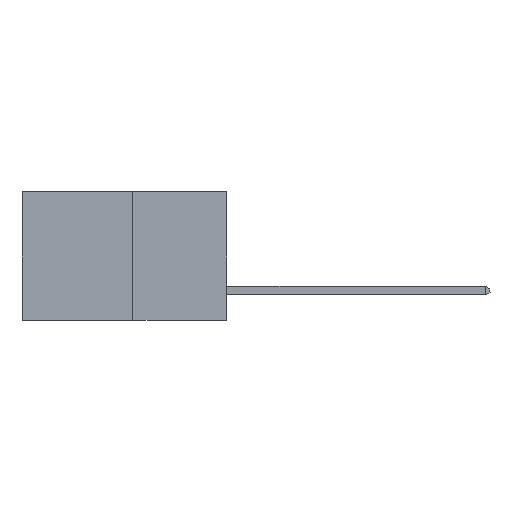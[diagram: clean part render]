
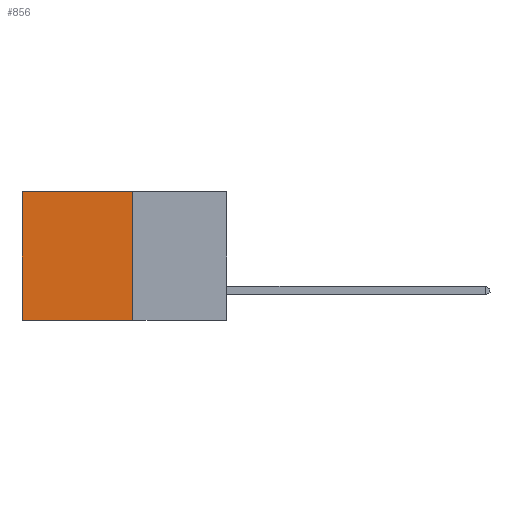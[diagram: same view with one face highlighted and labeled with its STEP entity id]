
A CAD part, left-side view. The second image highlights one B-rep face of the part: STEP entity #856.
In plain terms, the highlighted planar face has unit normal (-1, 0, 0).
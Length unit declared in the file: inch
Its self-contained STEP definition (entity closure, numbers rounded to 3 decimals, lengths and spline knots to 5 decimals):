
#461 = PLANE ( 'NONE',  #6389 ) ;
#600 = DIRECTION ( 'NONE',  ( 0., 0., -1. ) ) ;
#829 = DIRECTION ( 'NONE',  ( 0., 0., -1. ) ) ;
#856 = ADVANCED_FACE ( 'NONE', ( #1965 ), #461, .F. ) ;
#1067 = LINE ( 'NONE', #8534, #8472 ) ;
#1725 = VERTEX_POINT ( 'NONE', #8899 ) ;
#1933 = CARTESIAN_POINT ( 'NONE',  ( 0.277, 0.27, 0. ) ) ;
#1934 = ORIENTED_EDGE ( 'NONE', *, *, #11387, .T. ) ;
#1965 = FACE_OUTER_BOUND ( 'NONE', #11081, .T. ) ;
#2342 = VECTOR ( 'NONE', #3071, 39.37008 ) ;
#2908 = LINE ( 'NONE', #7714, #7548 ) ;
#3071 = DIRECTION ( 'NONE',  ( 0., 1., 0. ) ) ;
#4007 = CARTESIAN_POINT ( 'NONE',  ( 0.277, 0.27, 0. ) ) ;
#4614 = ORIENTED_EDGE ( 'NONE', *, *, #8416, .F. ) ;
#4676 = CARTESIAN_POINT ( 'NONE',  ( 0.277, 0.27, -0.37 ) ) ;
#5587 = DIRECTION ( 'NONE',  ( 0., 0., -1. ) ) ;
#6389 = AXIS2_PLACEMENT_3D ( 'NONE', #8666, #8728, #600 ) ;
#6515 = EDGE_CURVE ( 'NONE', #9696, #1725, #11638, .T. ) ;
#6874 = CARTESIAN_POINT ( 'NONE',  ( 0.277, 0.59, -0.37 ) ) ;
#7103 = LINE ( 'NONE', #1933, #2342 ) ;
#7548 = VECTOR ( 'NONE', #10431, 39.37008 ) ;
#7694 = VECTOR ( 'NONE', #5587, 39.37008 ) ;
#7714 = CARTESIAN_POINT ( 'NONE',  ( 0.277, 0.27, -0.37 ) ) ;
#8416 = EDGE_CURVE ( 'NONE', #1725, #9251, #2908, .T. ) ;
#8472 = VECTOR ( 'NONE', #829, 39.37008 ) ;
#8534 = CARTESIAN_POINT ( 'NONE',  ( 0.277, 0.59, -0.37 ) ) ;
#8666 = CARTESIAN_POINT ( 'NONE',  ( 0.277, 0.27, -0.37 ) ) ;
#8728 = DIRECTION ( 'NONE',  ( 1., 0., 0. ) ) ;
#8785 = CARTESIAN_POINT ( 'NONE',  ( 0.277, 0.59, 0. ) ) ;
#8899 = CARTESIAN_POINT ( 'NONE',  ( 0.277, 0.27, -0.37 ) ) ;
#9123 = EDGE_CURVE ( 'NONE', #9696, #12307, #7103, .T. ) ;
#9251 = VERTEX_POINT ( 'NONE', #6874 ) ;
#9416 = ORIENTED_EDGE ( 'NONE', *, *, #6515, .F. ) ;
#9696 = VERTEX_POINT ( 'NONE', #4007 ) ;
#10431 = DIRECTION ( 'NONE',  ( 0., 1., 0. ) ) ;
#11081 = EDGE_LOOP ( 'NONE', ( #1934, #4614, #9416, #11834 ) ) ;
#11387 = EDGE_CURVE ( 'NONE', #12307, #9251, #1067, .T. ) ;
#11638 = LINE ( 'NONE', #4676, #7694 ) ;
#11834 = ORIENTED_EDGE ( 'NONE', *, *, #9123, .T. ) ;
#12307 = VERTEX_POINT ( 'NONE', #8785 ) ;
